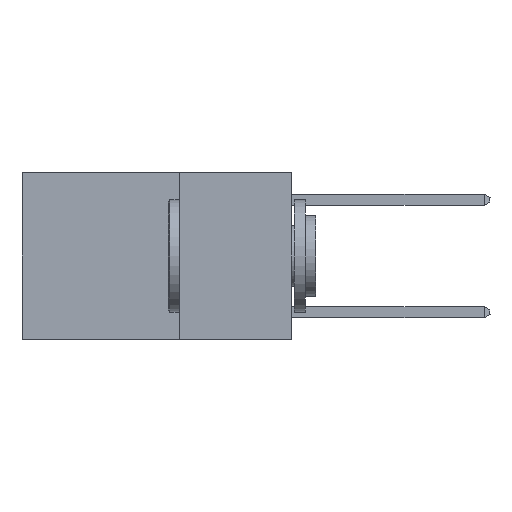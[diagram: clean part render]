
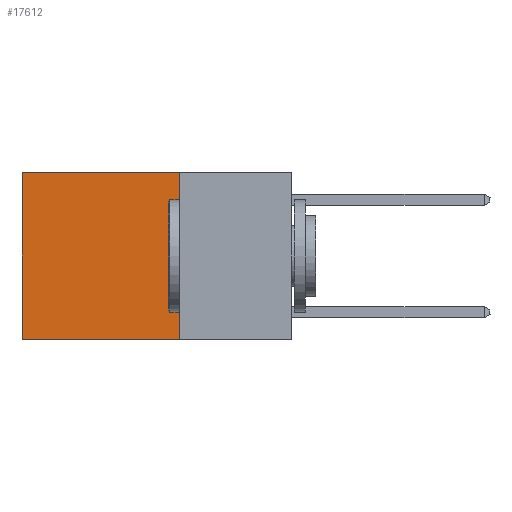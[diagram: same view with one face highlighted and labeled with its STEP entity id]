
A CAD part, left-side view. The second image highlights one B-rep face of the part: STEP entity #17612.
In plain terms, the highlighted planar face has unit normal (-1, 0, 0).
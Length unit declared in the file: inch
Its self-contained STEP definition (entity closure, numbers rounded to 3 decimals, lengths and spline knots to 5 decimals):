
#783 = EDGE_CURVE ( 'NONE', #15543, #6441, #4652, .T. ) ;
#1742 = CARTESIAN_POINT ( 'NONE',  ( 0.2625, 0.25, 0. ) ) ;
#3238 = EDGE_CURVE ( 'NONE', #6441, #4352, #15882, .T. ) ;
#4065 = ORIENTED_EDGE ( 'NONE', *, *, #14712, .T. ) ;
#4352 = VERTEX_POINT ( 'NONE', #11622 ) ;
#4641 = DIRECTION ( 'NONE',  ( 0., 0., -1. ) ) ;
#4652 = LINE ( 'NONE', #6165, #12347 ) ;
#5211 = ORIENTED_EDGE ( 'NONE', *, *, #783, .F. ) ;
#6069 = DIRECTION ( 'NONE',  ( 0., 0., -1. ) ) ;
#6155 = ORIENTED_EDGE ( 'NONE', *, *, #3238, .F. ) ;
#6165 = CARTESIAN_POINT ( 'NONE',  ( 0.2625, 0.25, 0. ) ) ;
#6441 = VERTEX_POINT ( 'NONE', #8219 ) ;
#7355 = LINE ( 'NONE', #16248, #10326 ) ;
#7516 = AXIS2_PLACEMENT_3D ( 'NONE', #1742, #15234, #10541 ) ;
#8219 = CARTESIAN_POINT ( 'NONE',  ( 0.2625, 0.25, -0.37 ) ) ;
#8233 = VERTEX_POINT ( 'NONE', #9983 ) ;
#8308 = DIRECTION ( 'NONE',  ( 0., 1., 0. ) ) ;
#9151 = PLANE ( 'NONE',  #7516 ) ;
#9983 = CARTESIAN_POINT ( 'NONE',  ( 0.2625, 0.6, 0. ) ) ;
#10326 = VECTOR ( 'NONE', #13537, 39.37008 ) ;
#10401 = CARTESIAN_POINT ( 'NONE',  ( 0.2625, 0.25, 0. ) ) ;
#10478 = VECTOR ( 'NONE', #8308, 39.37008 ) ;
#10541 = DIRECTION ( 'NONE',  ( 0., 0., -1. ) ) ;
#10649 = LINE ( 'NONE', #15132, #13812 ) ;
#11622 = CARTESIAN_POINT ( 'NONE',  ( 0.2625, 0.6, -0.37 ) ) ;
#11895 = ORIENTED_EDGE ( 'NONE', *, *, #15906, .T. ) ;
#12347 = VECTOR ( 'NONE', #6069, 39.37008 ) ;
#13537 = DIRECTION ( 'NONE',  ( 0., 1., 0. ) ) ;
#13812 = VECTOR ( 'NONE', #4641, 39.37008 ) ;
#14712 = EDGE_CURVE ( 'NONE', #8233, #4352, #10649, .T. ) ;
#15132 = CARTESIAN_POINT ( 'NONE',  ( 0.2625, 0.6, 0. ) ) ;
#15234 = DIRECTION ( 'NONE',  ( 1., 0., 0. ) ) ;
#15543 = VERTEX_POINT ( 'NONE', #10401 ) ;
#15882 = LINE ( 'NONE', #17009, #10478 ) ;
#15906 = EDGE_CURVE ( 'NONE', #15543, #8233, #7355, .T. ) ;
#16203 = EDGE_LOOP ( 'NONE', ( #4065, #6155, #5211, #11895 ) ) ;
#16248 = CARTESIAN_POINT ( 'NONE',  ( 0.2625, 0.25, 0. ) ) ;
#16741 = FACE_OUTER_BOUND ( 'NONE', #16203, .T. ) ;
#17009 = CARTESIAN_POINT ( 'NONE',  ( 0.2625, 0.25, -0.37 ) ) ;
#17612 = ADVANCED_FACE ( 'NONE', ( #16741 ), #9151, .F. ) ;
